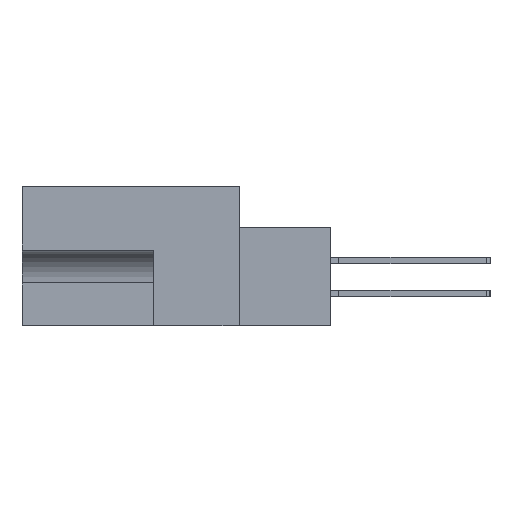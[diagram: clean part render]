
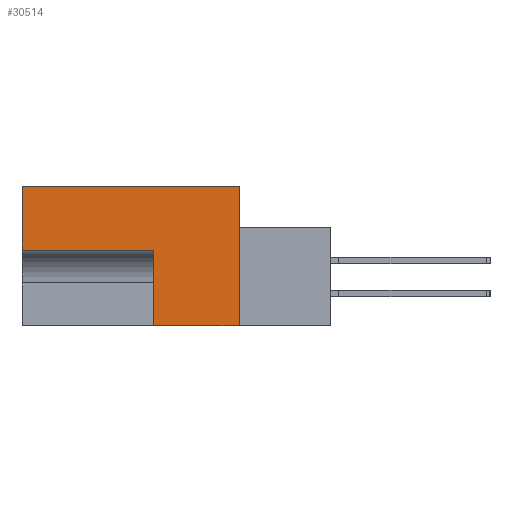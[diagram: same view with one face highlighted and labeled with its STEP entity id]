
A CAD part, left-side view. The second image highlights one B-rep face of the part: STEP entity #30514.
In plain terms, the highlighted planar face has unit normal (-1, 0, 0).
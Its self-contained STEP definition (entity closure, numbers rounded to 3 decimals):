
#2964 = LINE ( 'NONE', #6463, #40908 ) ;
#3171 = DIRECTION ( 'NONE',  ( 0., 1., 0. ) ) ;
#3410 = VECTOR ( 'NONE', #10421, 1000. ) ;
#4003 = LINE ( 'NONE', #39782, #39146 ) ;
#4059 = DIRECTION ( 'NONE',  ( 0., 0., -1. ) ) ;
#4854 = ORIENTED_EDGE ( 'NONE', *, *, #19541, .F. ) ;
#6463 = CARTESIAN_POINT ( 'NONE',  ( 0., -8.814, -13.487 ) ) ;
#7299 = ORIENTED_EDGE ( 'NONE', *, *, #34779, .F. ) ;
#7403 = CARTESIAN_POINT ( 'NONE',  ( 0., 0., 0. ) ) ;
#8112 = DIRECTION ( 'NONE',  ( 0., 1., 0. ) ) ;
#8551 = VECTOR ( 'NONE', #10863, 1000. ) ;
#9753 = EDGE_CURVE ( 'NONE', #21198, #43917, #4003, .T. ) ;
#10107 = CARTESIAN_POINT ( 'NONE',  ( 0., 20.955, -6.172 ) ) ;
#10421 = DIRECTION ( 'NONE',  ( 0., 0., -1. ) ) ;
#10612 = FACE_OUTER_BOUND ( 'NONE', #12756, .T. ) ;
#10863 = DIRECTION ( 'NONE',  ( 0., 0., 1. ) ) ;
#11252 = DIRECTION ( 'NONE',  ( 1., 0., 0. ) ) ;
#11337 = VECTOR ( 'NONE', #14096, 1000. ) ;
#12756 = EDGE_LOOP ( 'NONE', ( #4854, #44082, #7299, #41373, #29056, #23824 ) ) ;
#14096 = DIRECTION ( 'NONE',  ( 0., 0., 1. ) ) ;
#14688 = CARTESIAN_POINT ( 'NONE',  ( 0., 0., 0. ) ) ;
#19541 = EDGE_CURVE ( 'NONE', #36967, #40965, #2964, .T. ) ;
#19878 = CARTESIAN_POINT ( 'NONE',  ( 0., 11.506, 0. ) ) ;
#20025 = DIRECTION ( 'NONE',  ( 0., -1., 0. ) ) ;
#20825 = LINE ( 'NONE', #35267, #11337 ) ;
#21198 = VERTEX_POINT ( 'NONE', #29797 ) ;
#23824 = ORIENTED_EDGE ( 'NONE', *, *, #34889, .F. ) ;
#24097 = CARTESIAN_POINT ( 'NONE',  ( 0., 0., -13.487 ) ) ;
#24195 = VERTEX_POINT ( 'NONE', #7403 ) ;
#24322 = CARTESIAN_POINT ( 'NONE',  ( 0., 0., 0. ) ) ;
#25437 = PLANE ( 'NONE',  #39622 ) ;
#26413 = VECTOR ( 'NONE', #20025, 1000. ) ;
#27279 = CARTESIAN_POINT ( 'NONE',  ( 0., 8.255, -13.487 ) ) ;
#27530 = LINE ( 'NONE', #19878, #26413 ) ;
#29056 = ORIENTED_EDGE ( 'NONE', *, *, #9753, .F. ) ;
#29797 = CARTESIAN_POINT ( 'NONE',  ( 0., 8.255, -6.172 ) ) ;
#30514 = ADVANCED_FACE ( 'NONE', ( #10612 ), #25437, .F. ) ;
#34506 = EDGE_CURVE ( 'NONE', #43917, #36862, #41497, .T. ) ;
#34779 = EDGE_CURVE ( 'NONE', #36862, #24195, #27530, .T. ) ;
#34889 = EDGE_CURVE ( 'NONE', #40965, #21198, #20825, .T. ) ;
#35267 = CARTESIAN_POINT ( 'NONE',  ( 0., 8.255, -13.487 ) ) ;
#36862 = VERTEX_POINT ( 'NONE', #37323 ) ;
#36967 = VERTEX_POINT ( 'NONE', #24097 ) ;
#37323 = CARTESIAN_POINT ( 'NONE',  ( 0., 20.955, 0. ) ) ;
#39117 = LINE ( 'NONE', #24322, #3410 ) ;
#39146 = VECTOR ( 'NONE', #8112, 1000. ) ;
#39622 = AXIS2_PLACEMENT_3D ( 'NONE', #14688, #11252, #4059 ) ;
#39782 = CARTESIAN_POINT ( 'NONE',  ( 0., 8.255, -6.172 ) ) ;
#40908 = VECTOR ( 'NONE', #3171, 1000. ) ;
#40965 = VERTEX_POINT ( 'NONE', #27279 ) ;
#41090 = EDGE_CURVE ( 'NONE', #24195, #36967, #39117, .T. ) ;
#41373 = ORIENTED_EDGE ( 'NONE', *, *, #34506, .F. ) ;
#41497 = LINE ( 'NONE', #43167, #8551 ) ;
#43167 = CARTESIAN_POINT ( 'NONE',  ( 0., 20.955, -13.487 ) ) ;
#43917 = VERTEX_POINT ( 'NONE', #10107 ) ;
#44082 = ORIENTED_EDGE ( 'NONE', *, *, #41090, .F. ) ;
